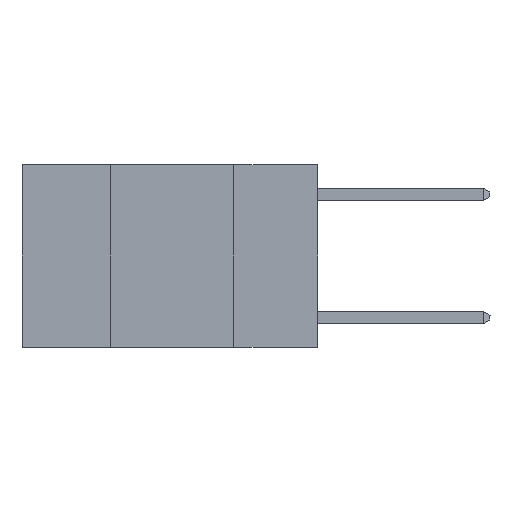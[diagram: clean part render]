
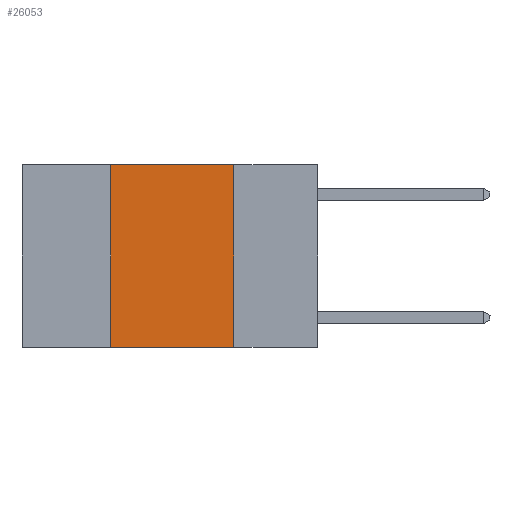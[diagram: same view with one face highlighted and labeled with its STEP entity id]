
A CAD part, left-side view. The second image highlights one B-rep face of the part: STEP entity #26053.
In plain terms, the highlighted planar face has unit normal (-1, 0, 0).
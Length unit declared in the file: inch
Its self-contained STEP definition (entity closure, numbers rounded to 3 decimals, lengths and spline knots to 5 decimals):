
#28 = PLANE ( 'NONE',  #21134 ) ;
#1192 = CARTESIAN_POINT ( 'NONE',  ( 0., 0.17, 0. ) ) ;
#2489 = VERTEX_POINT ( 'NONE', #9178 ) ;
#2626 = LINE ( 'NONE', #22440, #25599 ) ;
#5413 = ORIENTED_EDGE ( 'NONE', *, *, #13697, .T. ) ;
#5620 = EDGE_CURVE ( 'NONE', #2489, #8951, #15180, .T. ) ;
#5995 = DIRECTION ( 'NONE',  ( 0., 0., 1. ) ) ;
#6126 = DIRECTION ( 'NONE',  ( 0., -1., 0. ) ) ;
#6814 = DIRECTION ( 'NONE',  ( 1., 0., 0. ) ) ;
#8380 = CARTESIAN_POINT ( 'NONE',  ( 0., 0.6, -0.37 ) ) ;
#8951 = VERTEX_POINT ( 'NONE', #28069 ) ;
#9121 = DIRECTION ( 'NONE',  ( 0., -1., 0. ) ) ;
#9178 = CARTESIAN_POINT ( 'NONE',  ( 0., 0.42, -0.37 ) ) ;
#10134 = DIRECTION ( 'NONE',  ( 0., 0., -1. ) ) ;
#11649 = EDGE_CURVE ( 'NONE', #18377, #17026, #16561, .T. ) ;
#13697 = EDGE_CURVE ( 'NONE', #2489, #17026, #16150, .T. ) ;
#13836 = ORIENTED_EDGE ( 'NONE', *, *, #11649, .F. ) ;
#14465 = VECTOR ( 'NONE', #5995, 39.37008 ) ;
#15180 = LINE ( 'NONE', #19388, #14465 ) ;
#16150 = LINE ( 'NONE', #8380, #27130 ) ;
#16467 = EDGE_LOOP ( 'NONE', ( #13836, #18704, #27295, #5413 ) ) ;
#16561 = LINE ( 'NONE', #1192, #21740 ) ;
#16562 = EDGE_CURVE ( 'NONE', #8951, #18377, #2626, .T. ) ;
#17026 = VERTEX_POINT ( 'NONE', #18072 ) ;
#18072 = CARTESIAN_POINT ( 'NONE',  ( 0., 0.17, -0.37 ) ) ;
#18377 = VERTEX_POINT ( 'NONE', #24494 ) ;
#18704 = ORIENTED_EDGE ( 'NONE', *, *, #16562, .F. ) ;
#19388 = CARTESIAN_POINT ( 'NONE',  ( 0., 0.42, 0. ) ) ;
#20171 = CARTESIAN_POINT ( 'NONE',  ( 0., 0.6, 0. ) ) ;
#21134 = AXIS2_PLACEMENT_3D ( 'NONE', #20171, #6814, #22385 ) ;
#21740 = VECTOR ( 'NONE', #10134, 39.37008 ) ;
#22385 = DIRECTION ( 'NONE',  ( 0., 0., -1. ) ) ;
#22440 = CARTESIAN_POINT ( 'NONE',  ( 0., 0.6, 0. ) ) ;
#24494 = CARTESIAN_POINT ( 'NONE',  ( 0., 0.17, 0. ) ) ;
#25599 = VECTOR ( 'NONE', #9121, 39.37008 ) ;
#26053 = ADVANCED_FACE ( 'NONE', ( #26539 ), #28, .F. ) ;
#26539 = FACE_OUTER_BOUND ( 'NONE', #16467, .T. ) ;
#27130 = VECTOR ( 'NONE', #6126, 39.37008 ) ;
#27295 = ORIENTED_EDGE ( 'NONE', *, *, #5620, .F. ) ;
#28069 = CARTESIAN_POINT ( 'NONE',  ( 0., 0.42, 0. ) ) ;
